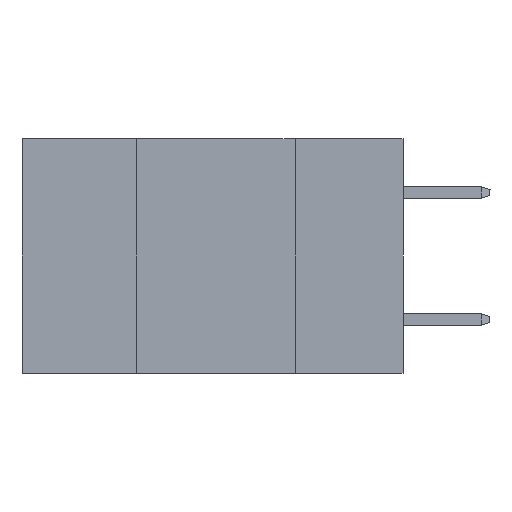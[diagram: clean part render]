
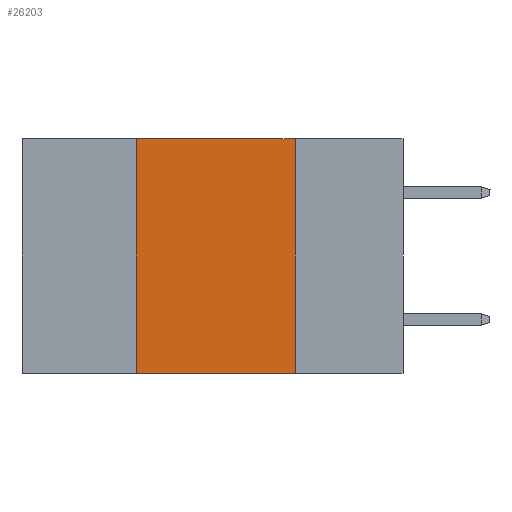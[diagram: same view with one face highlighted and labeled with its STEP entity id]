
A CAD part, left-side view. The second image highlights one B-rep face of the part: STEP entity #26203.
In plain terms, the highlighted planar face has unit normal (-1, 0, 0).
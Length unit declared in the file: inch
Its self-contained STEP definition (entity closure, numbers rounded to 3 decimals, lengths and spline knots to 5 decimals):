
#173 = LINE ( 'NONE', #28979, #1015 ) ;
#1015 = VECTOR ( 'NONE', #26870, 39.37008 ) ;
#1512 = VECTOR ( 'NONE', #10422, 39.37008 ) ;
#2116 = ORIENTED_EDGE ( 'NONE', *, *, #24673, .F. ) ;
#4201 = VERTEX_POINT ( 'NONE', #31198 ) ;
#4968 = CARTESIAN_POINT ( 'NONE',  ( 0., 0.17, 0. ) ) ;
#4992 = DIRECTION ( 'NONE',  ( 0., 0., -1. ) ) ;
#5755 = CARTESIAN_POINT ( 'NONE',  ( 0., 0.6, 0. ) ) ;
#6464 = CARTESIAN_POINT ( 'NONE',  ( 0., 0.42, 0. ) ) ;
#7266 = PLANE ( 'NONE',  #28912 ) ;
#7394 = DIRECTION ( 'NONE',  ( 0., -1., 0. ) ) ;
#8272 = VECTOR ( 'NONE', #7394, 39.37008 ) ;
#8963 = VERTEX_POINT ( 'NONE', #4968 ) ;
#10422 = DIRECTION ( 'NONE',  ( 0., -1., 0. ) ) ;
#11424 = VERTEX_POINT ( 'NONE', #20754 ) ;
#12384 = CARTESIAN_POINT ( 'NONE',  ( 0., 0.6, -0.37 ) ) ;
#14969 = FACE_OUTER_BOUND ( 'NONE', #23015, .T. ) ;
#15293 = CARTESIAN_POINT ( 'NONE',  ( 0., 0.42, 0. ) ) ;
#15751 = ORIENTED_EDGE ( 'NONE', *, *, #16022, .F. ) ;
#16022 = EDGE_CURVE ( 'NONE', #18648, #8963, #17989, .T. ) ;
#17989 = LINE ( 'NONE', #5755, #1512 ) ;
#18648 = VERTEX_POINT ( 'NONE', #15293 ) ;
#20754 = CARTESIAN_POINT ( 'NONE',  ( 0., 0.17, -0.37 ) ) ;
#21641 = EDGE_CURVE ( 'NONE', #8963, #11424, #173, .T. ) ;
#23015 = EDGE_LOOP ( 'NONE', ( #25783, #15751, #2116, #27564 ) ) ;
#23049 = EDGE_CURVE ( 'NONE', #4201, #11424, #29449, .T. ) ;
#23334 = LINE ( 'NONE', #6464, #25215 ) ;
#24673 = EDGE_CURVE ( 'NONE', #4201, #18648, #23334, .T. ) ;
#25215 = VECTOR ( 'NONE', #26087, 39.37008 ) ;
#25783 = ORIENTED_EDGE ( 'NONE', *, *, #21641, .F. ) ;
#26087 = DIRECTION ( 'NONE',  ( 0., 0., 1. ) ) ;
#26203 = ADVANCED_FACE ( 'NONE', ( #14969 ), #7266, .F. ) ;
#26870 = DIRECTION ( 'NONE',  ( 0., 0., -1. ) ) ;
#26892 = CARTESIAN_POINT ( 'NONE',  ( 0., 0.6, 0. ) ) ;
#27051 = DIRECTION ( 'NONE',  ( 1., 0., 0. ) ) ;
#27564 = ORIENTED_EDGE ( 'NONE', *, *, #23049, .T. ) ;
#28912 = AXIS2_PLACEMENT_3D ( 'NONE', #26892, #27051, #4992 ) ;
#28979 = CARTESIAN_POINT ( 'NONE',  ( 0., 0.17, 0. ) ) ;
#29449 = LINE ( 'NONE', #12384, #8272 ) ;
#31198 = CARTESIAN_POINT ( 'NONE',  ( 0., 0.42, -0.37 ) ) ;
